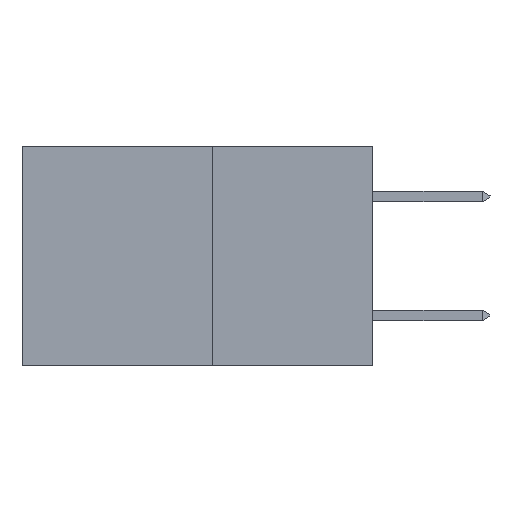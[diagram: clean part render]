
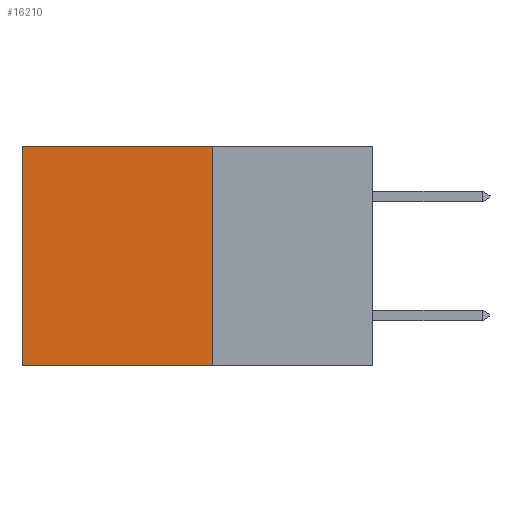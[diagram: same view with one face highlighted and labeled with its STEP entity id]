
A CAD part, left-side view. The second image highlights one B-rep face of the part: STEP entity #16210.
In plain terms, the highlighted planar face has unit normal (-1, 0, 0).
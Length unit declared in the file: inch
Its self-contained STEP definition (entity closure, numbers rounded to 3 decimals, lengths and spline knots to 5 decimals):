
#710 = VERTEX_POINT ( 'NONE', #24636 ) ;
#2910 = LINE ( 'NONE', #3702, #21293 ) ;
#3021 = ORIENTED_EDGE ( 'NONE', *, *, #27176, .T. ) ;
#3702 = CARTESIAN_POINT ( 'NONE',  ( 0.277, 0.59, -0.37 ) ) ;
#3729 = CARTESIAN_POINT ( 'NONE',  ( 0.277, 0.27, 0. ) ) ;
#3799 = LINE ( 'NONE', #25191, #29481 ) ;
#5327 = VERTEX_POINT ( 'NONE', #22168 ) ;
#7946 = VECTOR ( 'NONE', #21229, 39.37008 ) ;
#10365 = VECTOR ( 'NONE', #25955, 39.37008 ) ;
#10770 = DIRECTION ( 'NONE',  ( 1., 0., 0. ) ) ;
#11159 = LINE ( 'NONE', #23475, #10365 ) ;
#11828 = VERTEX_POINT ( 'NONE', #18548 ) ;
#12730 = ORIENTED_EDGE ( 'NONE', *, *, #22025, .F. ) ;
#13808 = LINE ( 'NONE', #3729, #7946 ) ;
#16210 = ADVANCED_FACE ( 'NONE', ( #30408 ), #18185, .F. ) ;
#16407 = ORIENTED_EDGE ( 'NONE', *, *, #28540, .T. ) ;
#17719 = CARTESIAN_POINT ( 'NONE',  ( 0.277, 0.27, -0.37 ) ) ;
#17882 = EDGE_LOOP ( 'NONE', ( #3021, #21484, #12730, #16407 ) ) ;
#18185 = PLANE ( 'NONE',  #29208 ) ;
#18548 = CARTESIAN_POINT ( 'NONE',  ( 0.277, 0.27, 0. ) ) ;
#20318 = DIRECTION ( 'NONE',  ( 0., 0., -1. ) ) ;
#21229 = DIRECTION ( 'NONE',  ( 0., 1., 0. ) ) ;
#21293 = VECTOR ( 'NONE', #28587, 39.37008 ) ;
#21484 = ORIENTED_EDGE ( 'NONE', *, *, #27099, .F. ) ;
#22025 = EDGE_CURVE ( 'NONE', #11828, #29784, #3799, .T. ) ;
#22168 = CARTESIAN_POINT ( 'NONE',  ( 0.277, 0.59, -0.37 ) ) ;
#23184 = CARTESIAN_POINT ( 'NONE',  ( 0.277, 0.27, -0.37 ) ) ;
#23475 = CARTESIAN_POINT ( 'NONE',  ( 0.277, 0.27, -0.37 ) ) ;
#24636 = CARTESIAN_POINT ( 'NONE',  ( 0.277, 0.59, 0. ) ) ;
#25191 = CARTESIAN_POINT ( 'NONE',  ( 0.277, 0.27, -0.37 ) ) ;
#25955 = DIRECTION ( 'NONE',  ( 0., 1., 0. ) ) ;
#27099 = EDGE_CURVE ( 'NONE', #29784, #5327, #11159, .T. ) ;
#27176 = EDGE_CURVE ( 'NONE', #710, #5327, #2910, .T. ) ;
#28114 = DIRECTION ( 'NONE',  ( 0., 0., -1. ) ) ;
#28540 = EDGE_CURVE ( 'NONE', #11828, #710, #13808, .T. ) ;
#28587 = DIRECTION ( 'NONE',  ( 0., 0., -1. ) ) ;
#29208 = AXIS2_PLACEMENT_3D ( 'NONE', #23184, #10770, #28114 ) ;
#29481 = VECTOR ( 'NONE', #20318, 39.37008 ) ;
#29784 = VERTEX_POINT ( 'NONE', #17719 ) ;
#30408 = FACE_OUTER_BOUND ( 'NONE', #17882, .T. ) ;
